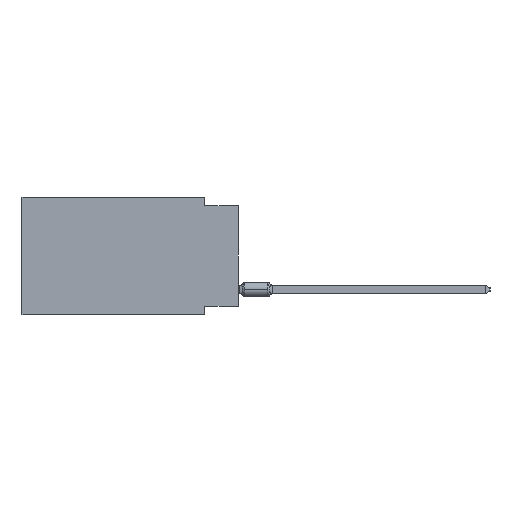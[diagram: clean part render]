
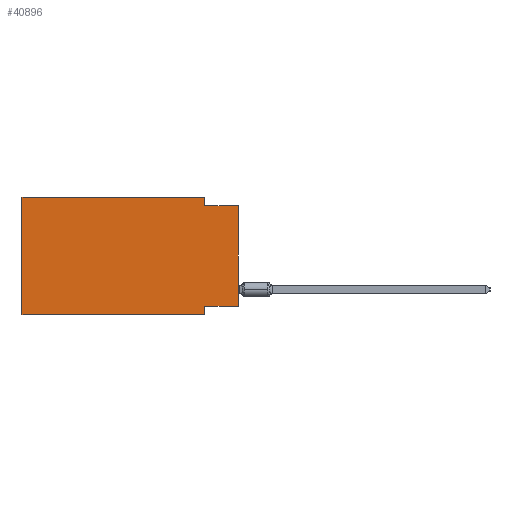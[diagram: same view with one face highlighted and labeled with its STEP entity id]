
A CAD part, left-side view. The second image highlights one B-rep face of the part: STEP entity #40896.
In plain terms, the highlighted planar face has unit normal (-1, 0, 0).
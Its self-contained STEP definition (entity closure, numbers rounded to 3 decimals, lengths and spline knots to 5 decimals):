
#1077 = CARTESIAN_POINT ( 'NONE',  ( 0., 0.645, 0. ) ) ;
#3588 = VERTEX_POINT ( 'NONE', #25350 ) ;
#6740 = ORIENTED_EDGE ( 'NONE', *, *, #37119, .T. ) ;
#9915 = DIRECTION ( 'NONE',  ( 0., 0., -1. ) ) ;
#10226 = CARTESIAN_POINT ( 'NONE',  ( 0., 0.645, 0. ) ) ;
#11254 = DIRECTION ( 'NONE',  ( 0., 0., 1. ) ) ;
#14077 = DIRECTION ( 'NONE',  ( 0., -1., 0. ) ) ;
#17308 = VERTEX_POINT ( 'NONE', #83470 ) ;
#17780 = LINE ( 'NONE', #10226, #90201 ) ;
#20218 = VERTEX_POINT ( 'NONE', #86759 ) ;
#21635 = LINE ( 'NONE', #52385, #44545 ) ;
#22560 = CARTESIAN_POINT ( 'NONE',  ( 0., 0.1, -0.35 ) ) ;
#24036 = DIRECTION ( 'NONE',  ( 1., 0., 0. ) ) ;
#25035 = PLANE ( 'NONE',  #37178 ) ;
#25350 = CARTESIAN_POINT ( 'NONE',  ( 0., 0.1, -0.025 ) ) ;
#26879 = CARTESIAN_POINT ( 'NONE',  ( 0., 0.1, 0. ) ) ;
#27289 = DIRECTION ( 'NONE',  ( 0., -1., 0. ) ) ;
#28589 = EDGE_CURVE ( 'NONE', #53424, #3588, #65680, .T. ) ;
#29407 = ORIENTED_EDGE ( 'NONE', *, *, #46987, .T. ) ;
#31418 = VERTEX_POINT ( 'NONE', #81452 ) ;
#32096 = CARTESIAN_POINT ( 'NONE',  ( 0., 0.645, 0. ) ) ;
#34565 = VECTOR ( 'NONE', #74933, 39.37008 ) ;
#35423 = EDGE_LOOP ( 'NONE', ( #6740, #78785, #79980, #98411, #99254, #29407, #78437, #97333 ) ) ;
#35491 = LINE ( 'NONE', #65745, #41911 ) ;
#37119 = EDGE_CURVE ( 'NONE', #17308, #38566, #58627, .T. ) ;
#37178 = AXIS2_PLACEMENT_3D ( 'NONE', #32096, #24036, #9915 ) ;
#37435 = CARTESIAN_POINT ( 'NONE',  ( 0., 0., -0.025 ) ) ;
#38566 = VERTEX_POINT ( 'NONE', #37435 ) ;
#38682 = DIRECTION ( 'NONE',  ( 0., 0., -1. ) ) ;
#40896 = ADVANCED_FACE ( 'NONE', ( #48713 ), #25035, .F. ) ;
#41911 = VECTOR ( 'NONE', #57687, 39.37008 ) ;
#44545 = VECTOR ( 'NONE', #14077, 39.37008 ) ;
#44966 = CARTESIAN_POINT ( 'NONE',  ( 0., 0.1, 0. ) ) ;
#46987 = EDGE_CURVE ( 'NONE', #50598, #31418, #98627, .T. ) ;
#48713 = FACE_OUTER_BOUND ( 'NONE', #35423, .T. ) ;
#50598 = VERTEX_POINT ( 'NONE', #92139 ) ;
#51555 = CARTESIAN_POINT ( 'NONE',  ( 0., 0., 0. ) ) ;
#52330 = LINE ( 'NONE', #81215, #73325 ) ;
#52385 = CARTESIAN_POINT ( 'NONE',  ( 0., 0.645, 0. ) ) ;
#52712 = VECTOR ( 'NONE', #95434, 39.37008 ) ;
#53424 = VERTEX_POINT ( 'NONE', #44966 ) ;
#55474 = EDGE_CURVE ( 'NONE', #20218, #31418, #91605, .T. ) ;
#56247 = VECTOR ( 'NONE', #38682, 39.37008 ) ;
#57687 = DIRECTION ( 'NONE',  ( 0., 1., 0. ) ) ;
#58401 = EDGE_CURVE ( 'NONE', #50598, #86650, #17780, .T. ) ;
#58627 = LINE ( 'NONE', #51555, #92931 ) ;
#65028 = EDGE_CURVE ( 'NONE', #17308, #20218, #35491, .T. ) ;
#65680 = LINE ( 'NONE', #26879, #52712 ) ;
#65745 = CARTESIAN_POINT ( 'NONE',  ( 0., 0., -0.325 ) ) ;
#72936 = EDGE_CURVE ( 'NONE', #3588, #38566, #52330, .T. ) ;
#73325 = VECTOR ( 'NONE', #27289, 39.37008 ) ;
#74933 = DIRECTION ( 'NONE',  ( 0., -1., 0. ) ) ;
#75422 = CARTESIAN_POINT ( 'NONE',  ( 0., 0.645, -0.35 ) ) ;
#76138 = EDGE_CURVE ( 'NONE', #86650, #53424, #21635, .T. ) ;
#78271 = DIRECTION ( 'NONE',  ( 0., 0., 1. ) ) ;
#78437 = ORIENTED_EDGE ( 'NONE', *, *, #55474, .F. ) ;
#78785 = ORIENTED_EDGE ( 'NONE', *, *, #72936, .F. ) ;
#79980 = ORIENTED_EDGE ( 'NONE', *, *, #28589, .F. ) ;
#81215 = CARTESIAN_POINT ( 'NONE',  ( 0., 0., -0.025 ) ) ;
#81452 = CARTESIAN_POINT ( 'NONE',  ( 0., 0.1, -0.35 ) ) ;
#83470 = CARTESIAN_POINT ( 'NONE',  ( 0., 0., -0.325 ) ) ;
#86650 = VERTEX_POINT ( 'NONE', #1077 ) ;
#86759 = CARTESIAN_POINT ( 'NONE',  ( 0., 0.1, -0.325 ) ) ;
#90201 = VECTOR ( 'NONE', #78271, 39.37008 ) ;
#91605 = LINE ( 'NONE', #22560, #56247 ) ;
#92139 = CARTESIAN_POINT ( 'NONE',  ( 0., 0.645, -0.35 ) ) ;
#92931 = VECTOR ( 'NONE', #11254, 39.37008 ) ;
#95434 = DIRECTION ( 'NONE',  ( 0., 0., -1. ) ) ;
#97333 = ORIENTED_EDGE ( 'NONE', *, *, #65028, .F. ) ;
#98411 = ORIENTED_EDGE ( 'NONE', *, *, #76138, .F. ) ;
#98627 = LINE ( 'NONE', #75422, #34565 ) ;
#99254 = ORIENTED_EDGE ( 'NONE', *, *, #58401, .F. ) ;
